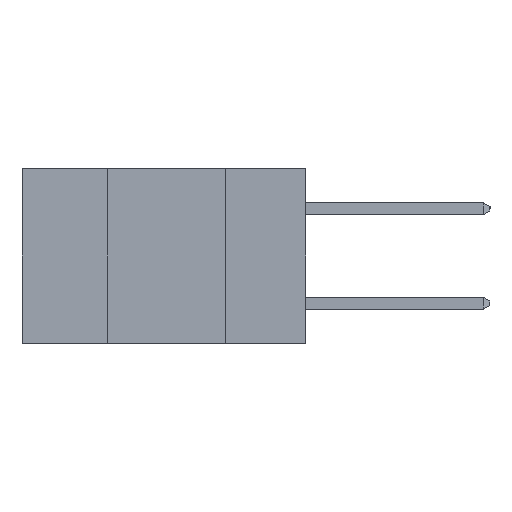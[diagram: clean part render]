
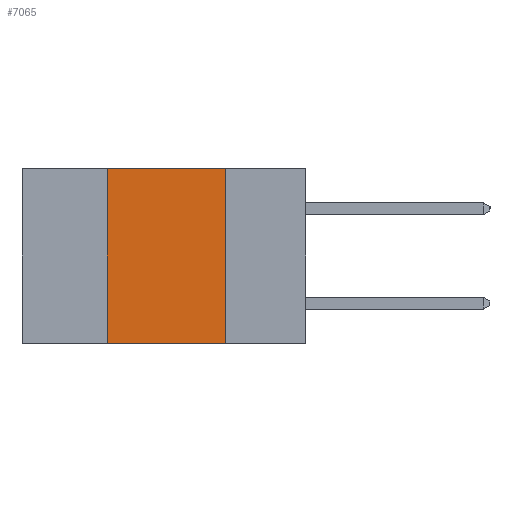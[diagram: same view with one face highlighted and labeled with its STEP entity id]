
A CAD part, left-side view. The second image highlights one B-rep face of the part: STEP entity #7065.
In plain terms, the highlighted planar face has unit normal (-1, 0, 0).
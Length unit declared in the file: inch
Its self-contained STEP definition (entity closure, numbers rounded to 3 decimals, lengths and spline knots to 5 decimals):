
#25 = EDGE_CURVE ( 'NONE', #13652, #9775, #11924, .T. ) ;
#454 = CARTESIAN_POINT ( 'NONE',  ( 0., 0.17, 0. ) ) ;
#479 = DIRECTION ( 'NONE',  ( 0., 0., -1. ) ) ;
#2885 = VECTOR ( 'NONE', #17915, 39.37008 ) ;
#2911 = EDGE_LOOP ( 'NONE', ( #18415, #14356, #7753, #8351 ) ) ;
#5802 = EDGE_CURVE ( 'NONE', #9775, #21629, #18051, .T. ) ;
#6156 = VECTOR ( 'NONE', #16243, 39.37008 ) ;
#6219 = CARTESIAN_POINT ( 'NONE',  ( 0., 0.6, 0. ) ) ;
#7065 = ADVANCED_FACE ( 'NONE', ( #17811 ), #23656, .F. ) ;
#7201 = CARTESIAN_POINT ( 'NONE',  ( 0., 0.42, -0.37 ) ) ;
#7753 = ORIENTED_EDGE ( 'NONE', *, *, #14380, .F. ) ;
#7994 = CARTESIAN_POINT ( 'NONE',  ( 0., 0.6, 0. ) ) ;
#8344 = LINE ( 'NONE', #21823, #6156 ) ;
#8351 = ORIENTED_EDGE ( 'NONE', *, *, #9873, .T. ) ;
#9316 = LINE ( 'NONE', #16958, #20948 ) ;
#9550 = DIRECTION ( 'NONE',  ( 0., 0., -1. ) ) ;
#9775 = VERTEX_POINT ( 'NONE', #454 ) ;
#9873 = EDGE_CURVE ( 'NONE', #10079, #21629, #8344, .T. ) ;
#10079 = VERTEX_POINT ( 'NONE', #7201 ) ;
#11924 = LINE ( 'NONE', #7994, #2885 ) ;
#13652 = VERTEX_POINT ( 'NONE', #21818 ) ;
#13991 = DIRECTION ( 'NONE',  ( 1., 0., 0. ) ) ;
#14356 = ORIENTED_EDGE ( 'NONE', *, *, #25, .F. ) ;
#14380 = EDGE_CURVE ( 'NONE', #10079, #13652, #9316, .T. ) ;
#14494 = CARTESIAN_POINT ( 'NONE',  ( 0., 0.17, -0.37 ) ) ;
#16243 = DIRECTION ( 'NONE',  ( 0., -1., 0. ) ) ;
#16958 = CARTESIAN_POINT ( 'NONE',  ( 0., 0.42, -0.37 ) ) ;
#17398 = AXIS2_PLACEMENT_3D ( 'NONE', #6219, #13991, #9550 ) ;
#17811 = FACE_OUTER_BOUND ( 'NONE', #2911, .T. ) ;
#17915 = DIRECTION ( 'NONE',  ( 0., -1., 0. ) ) ;
#18051 = LINE ( 'NONE', #14494, #20589 ) ;
#18415 = ORIENTED_EDGE ( 'NONE', *, *, #5802, .F. ) ;
#20589 = VECTOR ( 'NONE', #479, 39.37008 ) ;
#20948 = VECTOR ( 'NONE', #23044, 39.37008 ) ;
#21629 = VERTEX_POINT ( 'NONE', #23653 ) ;
#21818 = CARTESIAN_POINT ( 'NONE',  ( 0., 0.42, 0. ) ) ;
#21823 = CARTESIAN_POINT ( 'NONE',  ( 0., 0.6, -0.37 ) ) ;
#23044 = DIRECTION ( 'NONE',  ( 0., 0., 1. ) ) ;
#23653 = CARTESIAN_POINT ( 'NONE',  ( 0., 0.17, -0.37 ) ) ;
#23656 = PLANE ( 'NONE',  #17398 ) ;
